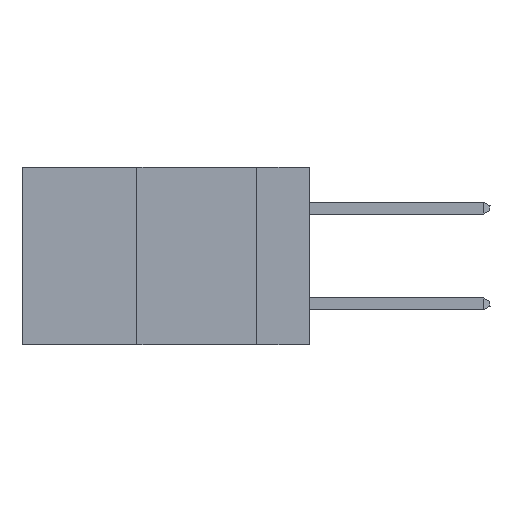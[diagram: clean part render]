
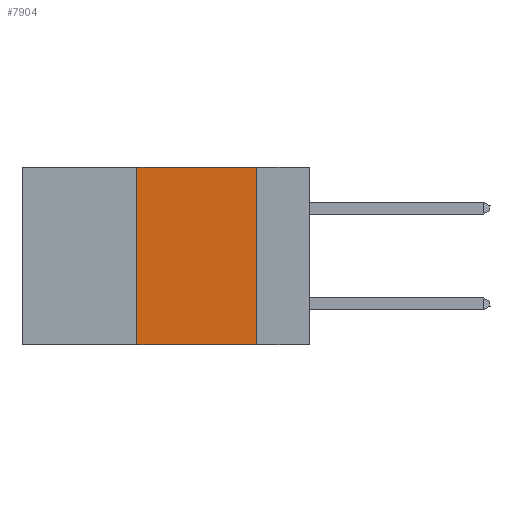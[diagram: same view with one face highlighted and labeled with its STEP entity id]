
A CAD part, left-side view. The second image highlights one B-rep face of the part: STEP entity #7904.
In plain terms, the highlighted planar face has unit normal (-1, 0, 0).
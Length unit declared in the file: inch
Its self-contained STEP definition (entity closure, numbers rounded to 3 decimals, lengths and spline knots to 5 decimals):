
#230 = EDGE_LOOP ( 'NONE', ( #25676, #17985, #28964, #24309 ) ) ;
#261 = DIRECTION ( 'NONE',  ( 0., 0., -1. ) ) ;
#1718 = VECTOR ( 'NONE', #30651, 39.37008 ) ;
#5234 = LINE ( 'NONE', #28031, #33705 ) ;
#7904 = ADVANCED_FACE ( 'NONE', ( #18128 ), #12794, .F. ) ;
#9631 = CARTESIAN_POINT ( 'NONE',  ( 0., 0.6, 0. ) ) ;
#12253 = VERTEX_POINT ( 'NONE', #28162 ) ;
#12454 = CARTESIAN_POINT ( 'NONE',  ( 0., 0.11, 0. ) ) ;
#12794 = PLANE ( 'NONE',  #26127 ) ;
#12997 = CARTESIAN_POINT ( 'NONE',  ( 0., 0.6, 0. ) ) ;
#14257 = VECTOR ( 'NONE', #20413, 39.37008 ) ;
#16128 = VECTOR ( 'NONE', #261, 39.37008 ) ;
#16149 = VERTEX_POINT ( 'NONE', #33770 ) ;
#16452 = CARTESIAN_POINT ( 'NONE',  ( 0., 0.11, 0. ) ) ;
#16869 = EDGE_CURVE ( 'NONE', #26889, #18744, #30372, .T. ) ;
#17985 = ORIENTED_EDGE ( 'NONE', *, *, #16869, .F. ) ;
#18128 = FACE_OUTER_BOUND ( 'NONE', #230, .T. ) ;
#18744 = VERTEX_POINT ( 'NONE', #12454 ) ;
#19480 = DIRECTION ( 'NONE',  ( 1., 0., 0. ) ) ;
#20413 = DIRECTION ( 'NONE',  ( 0., -1., 0. ) ) ;
#21580 = LINE ( 'NONE', #22443, #1718 ) ;
#22443 = CARTESIAN_POINT ( 'NONE',  ( 0., 0.6, -0.37 ) ) ;
#22460 = EDGE_CURVE ( 'NONE', #18744, #16149, #24176, .T. ) ;
#24176 = LINE ( 'NONE', #16452, #16128 ) ;
#24309 = ORIENTED_EDGE ( 'NONE', *, *, #29972, .T. ) ;
#25676 = ORIENTED_EDGE ( 'NONE', *, *, #22460, .F. ) ;
#26127 = AXIS2_PLACEMENT_3D ( 'NONE', #12997, #19480, #30723 ) ;
#26889 = VERTEX_POINT ( 'NONE', #29524 ) ;
#27899 = EDGE_CURVE ( 'NONE', #12253, #26889, #5234, .T. ) ;
#28031 = CARTESIAN_POINT ( 'NONE',  ( 0., 0.36, 0. ) ) ;
#28145 = DIRECTION ( 'NONE',  ( 0., 0., 1. ) ) ;
#28162 = CARTESIAN_POINT ( 'NONE',  ( 0., 0.36, -0.37 ) ) ;
#28964 = ORIENTED_EDGE ( 'NONE', *, *, #27899, .F. ) ;
#29524 = CARTESIAN_POINT ( 'NONE',  ( 0., 0.36, 0. ) ) ;
#29972 = EDGE_CURVE ( 'NONE', #12253, #16149, #21580, .T. ) ;
#30372 = LINE ( 'NONE', #9631, #14257 ) ;
#30651 = DIRECTION ( 'NONE',  ( 0., -1., 0. ) ) ;
#30723 = DIRECTION ( 'NONE',  ( 0., 0., -1. ) ) ;
#33705 = VECTOR ( 'NONE', #28145, 39.37008 ) ;
#33770 = CARTESIAN_POINT ( 'NONE',  ( 0., 0.11, -0.37 ) ) ;
